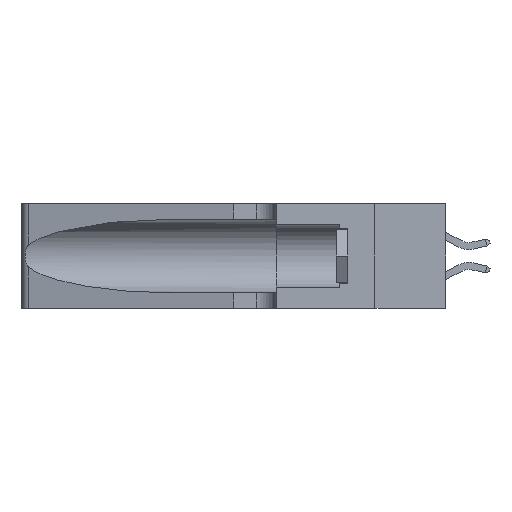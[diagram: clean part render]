
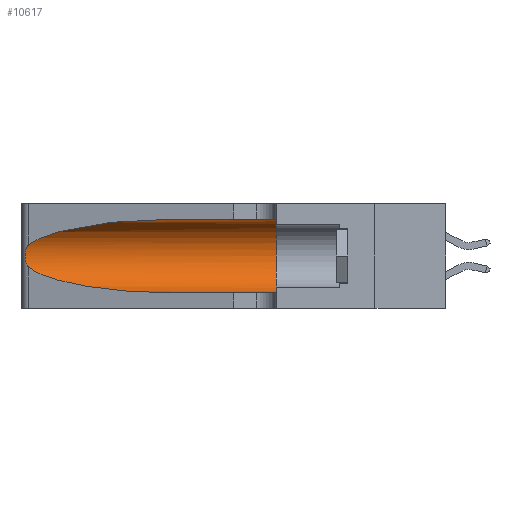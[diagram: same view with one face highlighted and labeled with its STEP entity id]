
A CAD part, left-side view. The second image highlights one B-rep face of the part: STEP entity #10617.
In plain terms, the highlighted cylindrical face has radius 3.308 mm (diameter 6.617 mm), a partial arc.
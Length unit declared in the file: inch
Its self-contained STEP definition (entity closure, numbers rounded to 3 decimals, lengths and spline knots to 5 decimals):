
#4 = CARTESIAN_POINT ( 'NONE',  ( 0.25487, 1.22718, 0.22369 ) ) ;
#269 = B_SPLINE_CURVE_WITH_KNOTS ( 'NONE', 3,
 ( #20131, #9836, #21865, #11651, #613, #13409, #2505, #15096, #4433, #16813, #6276, #18483, #8097, #20205 ),
 .UNSPECIFIED., .F., .F.,
 ( 4, 2, 2, 2, 2, 2, 4 ),
 ( 0., 0.00027, 0.00053, 0.00107, 0.0016, 0.00187, 0.00214 ),
 .UNSPECIFIED. ) ;
#613 = CARTESIAN_POINT ( 'NONE',  ( 0.25854, 1.2359, 0.20912 ) ) ;
#1051 =( BOUNDED_CURVE ( )  B_SPLINE_CURVE ( 3, ( #19590, #7439, #11092, #4 ),
 .UNSPECIFIED., .F., .F. ) 
 B_SPLINE_CURVE_WITH_KNOTS ( ( 4, 4 ),
 ( 1.5708, 2.84003 ),
 .UNSPECIFIED. ) 
 CURVE ( )  GEOMETRIC_REPRESENTATION_ITEM ( )  RATIONAL_B_SPLINE_CURVE ( ( 1., 0.87, 0.87, 1. ) ) 
 REPRESENTATION_ITEM ( '' )  );
#1235 = ORIENTED_EDGE ( 'NONE', *, *, #16208, .T. ) ;
#1636 =( BOUNDED_CURVE ( )  B_SPLINE_CURVE ( 3, ( #21612, #9581, #5945, #11376 ),
 .UNSPECIFIED., .F., .F. ) 
 B_SPLINE_CURVE_WITH_KNOTS ( ( 4, 4 ),
 ( 3.44316, 4.71239 ),
 .UNSPECIFIED. ) 
 CURVE ( )  GEOMETRIC_REPRESENTATION_ITEM ( )  RATIONAL_B_SPLINE_CURVE ( ( 1., 0.87, 0.87, 1. ) ) 
 REPRESENTATION_ITEM ( '' )  );
#2127 = ORIENTED_EDGE ( 'NONE', *, *, #12959, .F. ) ;
#2407 = CARTESIAN_POINT ( 'NONE',  ( 0.1305, 1.61858, 0.31525 ) ) ;
#2505 = CARTESIAN_POINT ( 'NONE',  ( 0.26075, 1.23896, 0.19203 ) ) ;
#2641 = CARTESIAN_POINT ( 'NONE',  ( 0.1305, 1.61858, 0.05475 ) ) ;
#3474 = EDGE_LOOP ( 'NONE', ( #22506, #12418, #19042, #1235, #2127, #7644 ) ) ;
#3970 = CARTESIAN_POINT ( 'NONE',  ( 0.1305, 0.35, 0.31525 ) ) ;
#4433 = CARTESIAN_POINT ( 'NONE',  ( 0.26017, 1.23833, 0.17102 ) ) ;
#4862 = CARTESIAN_POINT ( 'NONE',  ( 0.25487, 1.22718, 0.14631 ) ) ;
#5945 = CARTESIAN_POINT ( 'NONE',  ( 0.18966, 0.96281, 0.05475 ) ) ;
#6121 = VERTEX_POINT ( 'NONE', #20894 ) ;
#6276 = CARTESIAN_POINT ( 'NONE',  ( 0.25789, 1.23486, 0.15765 ) ) ;
#6363 = CIRCLE ( 'NONE', #19549, 0.13025 ) ;
#6387 = DIRECTION ( 'NONE',  ( 0., -1., 0. ) ) ;
#6463 = EDGE_CURVE ( 'NONE', #16732, #16018, #13844, .T. ) ;
#7198 = CARTESIAN_POINT ( 'NONE',  ( 0.1305, 0.35, 0.185 ) ) ;
#7439 = CARTESIAN_POINT ( 'NONE',  ( 0.18966, 0.96281, 0.31525 ) ) ;
#7644 = ORIENTED_EDGE ( 'NONE', *, *, #6463, .F. ) ;
#8097 = CARTESIAN_POINT ( 'NONE',  ( 0.25555, 1.22993, 0.14849 ) ) ;
#8876 = CARTESIAN_POINT ( 'NONE',  ( 0.25487, 1.22718, 0.22369 ) ) ;
#8887 = EDGE_CURVE ( 'NONE', #12778, #11248, #1636, .T. ) ;
#9038 = DIRECTION ( 'NONE',  ( 0., -1., 0. ) ) ;
#9048 = DIRECTION ( 'NONE',  ( 0., 0., 1. ) ) ;
#9457 = CARTESIAN_POINT ( 'NONE',  ( 0.1305, 0.72297, 0.31525 ) ) ;
#9581 = CARTESIAN_POINT ( 'NONE',  ( 0.2373, 1.15595, 0.08982 ) ) ;
#9836 = CARTESIAN_POINT ( 'NONE',  ( 0.25555, 1.22994, 0.2215 ) ) ;
#9890 = AXIS2_PLACEMENT_3D ( 'NONE', #17591, #9038, #10844 ) ;
#10544 = VERTEX_POINT ( 'NONE', #8876 ) ;
#10617 = ADVANCED_FACE ( 'NONE', ( #11053 ), #17983, .F. ) ;
#10683 = EDGE_CURVE ( 'NONE', #16732, #10544, #1051, .T. ) ;
#10742 = CARTESIAN_POINT ( 'NONE',  ( 0.1305, 0.72297, 0.05475 ) ) ;
#10844 = DIRECTION ( 'NONE',  ( 0., 0., -1. ) ) ;
#11053 = FACE_OUTER_BOUND ( 'NONE', #3474, .T. ) ;
#11092 = CARTESIAN_POINT ( 'NONE',  ( 0.2373, 1.15595, 0.28018 ) ) ;
#11248 = VERTEX_POINT ( 'NONE', #10742 ) ;
#11288 = LINE ( 'NONE', #2641, #19823 ) ;
#11376 = CARTESIAN_POINT ( 'NONE',  ( 0.1305, 0.72297, 0.05475 ) ) ;
#11641 = DIRECTION ( 'NONE',  ( 0., -1., 0. ) ) ;
#11651 = CARTESIAN_POINT ( 'NONE',  ( 0.25787, 1.23484, 0.2124 ) ) ;
#12418 = ORIENTED_EDGE ( 'NONE', *, *, #13149, .T. ) ;
#12778 = VERTEX_POINT ( 'NONE', #4862 ) ;
#12959 = EDGE_CURVE ( 'NONE', #16018, #6121, #6363, .T. ) ;
#13149 = EDGE_CURVE ( 'NONE', #10544, #12778, #269, .T. ) ;
#13409 = CARTESIAN_POINT ( 'NONE',  ( 0.26018, 1.23835, 0.19895 ) ) ;
#13844 = LINE ( 'NONE', #2407, #17279 ) ;
#15096 = CARTESIAN_POINT ( 'NONE',  ( 0.26075, 1.23896, 0.178 ) ) ;
#16018 = VERTEX_POINT ( 'NONE', #3970 ) ;
#16208 = EDGE_CURVE ( 'NONE', #11248, #6121, #11288, .T. ) ;
#16732 = VERTEX_POINT ( 'NONE', #9457 ) ;
#16813 = CARTESIAN_POINT ( 'NONE',  ( 0.25856, 1.23593, 0.16098 ) ) ;
#17279 = VECTOR ( 'NONE', #11641, 39.37008 ) ;
#17591 = CARTESIAN_POINT ( 'NONE',  ( 0.1305, 1.61858, 0.185 ) ) ;
#17983 = CYLINDRICAL_SURFACE ( 'NONE', #9890, 0.13025 ) ;
#18483 = CARTESIAN_POINT ( 'NONE',  ( 0.25639, 1.23186, 0.15144 ) ) ;
#19042 = ORIENTED_EDGE ( 'NONE', *, *, #8887, .T. ) ;
#19368 = DIRECTION ( 'NONE',  ( 0., 1., 0. ) ) ;
#19549 = AXIS2_PLACEMENT_3D ( 'NONE', #7198, #19368, #9048 ) ;
#19590 = CARTESIAN_POINT ( 'NONE',  ( 0.1305, 0.72297, 0.31525 ) ) ;
#19823 = VECTOR ( 'NONE', #6387, 39.37008 ) ;
#20131 = CARTESIAN_POINT ( 'NONE',  ( 0.25487, 1.22718, 0.22369 ) ) ;
#20205 = CARTESIAN_POINT ( 'NONE',  ( 0.25487, 1.22718, 0.14631 ) ) ;
#20894 = CARTESIAN_POINT ( 'NONE',  ( 0.1305, 0.35, 0.05475 ) ) ;
#21612 = CARTESIAN_POINT ( 'NONE',  ( 0.25487, 1.22718, 0.14631 ) ) ;
#21865 = CARTESIAN_POINT ( 'NONE',  ( 0.25639, 1.23184, 0.21858 ) ) ;
#22506 = ORIENTED_EDGE ( 'NONE', *, *, #10683, .T. ) ;
